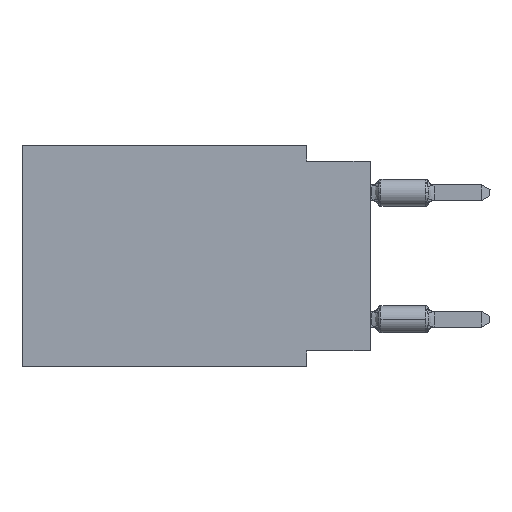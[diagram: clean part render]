
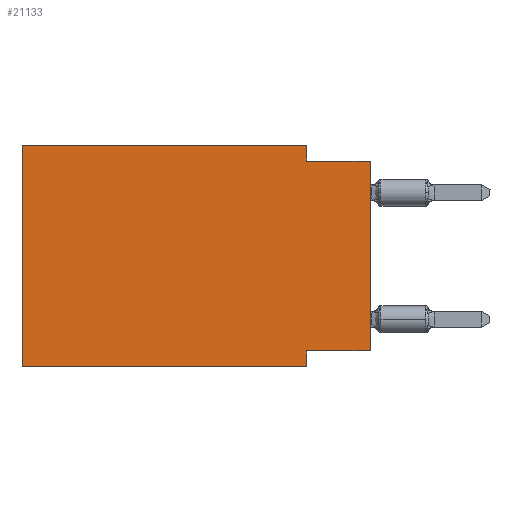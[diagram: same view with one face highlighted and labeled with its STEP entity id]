
A CAD part, left-side view. The second image highlights one B-rep face of the part: STEP entity #21133.
In plain terms, the highlighted planar face has unit normal (-1, 0, 0).
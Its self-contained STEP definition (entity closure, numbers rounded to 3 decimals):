
#241 = EDGE_CURVE ( 'NONE', #34653, #24544, #29616, .T. ) ;
#618 = CARTESIAN_POINT ( 'NONE',  ( 0., 13.97, -8.89 ) ) ;
#690 = DIRECTION ( 'NONE',  ( 0., -1., 0. ) ) ;
#969 = DIRECTION ( 'NONE',  ( 0., 0., -1. ) ) ;
#2252 = CARTESIAN_POINT ( 'NONE',  ( 0., 2.54, 0. ) ) ;
#2340 = EDGE_CURVE ( 'NONE', #28692, #20723, #17113, .T. ) ;
#2388 = CARTESIAN_POINT ( 'NONE',  ( 0., 13.97, 0. ) ) ;
#2437 = VERTEX_POINT ( 'NONE', #8050 ) ;
#2706 = VECTOR ( 'NONE', #32780, 1000. ) ;
#3138 = LINE ( 'NONE', #618, #26369 ) ;
#3163 = ORIENTED_EDGE ( 'NONE', *, *, #15992, .F. ) ;
#3321 = CARTESIAN_POINT ( 'NONE',  ( 0., 13.97, 0. ) ) ;
#4122 = AXIS2_PLACEMENT_3D ( 'NONE', #15893, #6894, #10316 ) ;
#4881 = CARTESIAN_POINT ( 'NONE',  ( 0., 13.97, 0. ) ) ;
#5258 = CARTESIAN_POINT ( 'NONE',  ( 0., 2.54, -0.635 ) ) ;
#6297 = CARTESIAN_POINT ( 'NONE',  ( 0., 2.54, -8.255 ) ) ;
#6429 = VECTOR ( 'NONE', #21536, 1000. ) ;
#6894 = DIRECTION ( 'NONE',  ( 1., 0., 0. ) ) ;
#7183 = VECTOR ( 'NONE', #969, 1000. ) ;
#7878 = LINE ( 'NONE', #2252, #2706 ) ;
#8050 = CARTESIAN_POINT ( 'NONE',  ( 0., 0., -8.255 ) ) ;
#8384 = VECTOR ( 'NONE', #26746, 1000. ) ;
#10316 = DIRECTION ( 'NONE',  ( 0., 0., -1. ) ) ;
#10370 = CARTESIAN_POINT ( 'NONE',  ( 0., 0., -8.255 ) ) ;
#10585 = CARTESIAN_POINT ( 'NONE',  ( 0., 2.54, -8.89 ) ) ;
#11467 = EDGE_CURVE ( 'NONE', #20013, #22165, #28789, .T. ) ;
#12053 = EDGE_CURVE ( 'NONE', #2437, #20723, #32335, .T. ) ;
#12486 = PLANE ( 'NONE',  #4122 ) ;
#12801 = ORIENTED_EDGE ( 'NONE', *, *, #241, .F. ) ;
#12854 = EDGE_CURVE ( 'NONE', #2437, #20013, #18299, .T. ) ;
#12998 = CARTESIAN_POINT ( 'NONE',  ( 0., 0., -0.635 ) ) ;
#14737 = ORIENTED_EDGE ( 'NONE', *, *, #34406, .T. ) ;
#15375 = VECTOR ( 'NONE', #16526, 1000. ) ;
#15893 = CARTESIAN_POINT ( 'NONE',  ( 0., 13.97, 0. ) ) ;
#15992 = EDGE_CURVE ( 'NONE', #29948, #34653, #22479, .T. ) ;
#16526 = DIRECTION ( 'NONE',  ( 0., 0., 1. ) ) ;
#16548 = ORIENTED_EDGE ( 'NONE', *, *, #2340, .F. ) ;
#17113 = LINE ( 'NONE', #23250, #28188 ) ;
#18299 = LINE ( 'NONE', #10370, #6429 ) ;
#20013 = VERTEX_POINT ( 'NONE', #6297 ) ;
#20466 = CARTESIAN_POINT ( 'NONE',  ( 0., 2.54, -8.89 ) ) ;
#20723 = VERTEX_POINT ( 'NONE', #12998 ) ;
#21133 = ADVANCED_FACE ( 'NONE', ( #34695 ), #12486, .F. ) ;
#21536 = DIRECTION ( 'NONE',  ( 0., 1., 0. ) ) ;
#22165 = VERTEX_POINT ( 'NONE', #10585 ) ;
#22479 = LINE ( 'NONE', #3321, #15375 ) ;
#22510 = ORIENTED_EDGE ( 'NONE', *, *, #12854, .F. ) ;
#23250 = CARTESIAN_POINT ( 'NONE',  ( 0., 0., -0.635 ) ) ;
#23537 = VECTOR ( 'NONE', #32503, 1000. ) ;
#24210 = CARTESIAN_POINT ( 'NONE',  ( 0., 0., 0. ) ) ;
#24488 = ORIENTED_EDGE ( 'NONE', *, *, #12053, .T. ) ;
#24544 = VERTEX_POINT ( 'NONE', #29024 ) ;
#24953 = ORIENTED_EDGE ( 'NONE', *, *, #11467, .F. ) ;
#26369 = VECTOR ( 'NONE', #30247, 1000. ) ;
#26746 = DIRECTION ( 'NONE',  ( 0., 0., 1. ) ) ;
#28188 = VECTOR ( 'NONE', #690, 1000. ) ;
#28692 = VERTEX_POINT ( 'NONE', #5258 ) ;
#28789 = LINE ( 'NONE', #20466, #7183 ) ;
#29024 = CARTESIAN_POINT ( 'NONE',  ( 0., 2.54, 0. ) ) ;
#29616 = LINE ( 'NONE', #4881, #23537 ) ;
#29948 = VERTEX_POINT ( 'NONE', #34495 ) ;
#30097 = EDGE_LOOP ( 'NONE', ( #24488, #16548, #30686, #12801, #3163, #14737, #24953, #22510 ) ) ;
#30247 = DIRECTION ( 'NONE',  ( 0., -1., 0. ) ) ;
#30686 = ORIENTED_EDGE ( 'NONE', *, *, #34294, .F. ) ;
#32335 = LINE ( 'NONE', #24210, #8384 ) ;
#32503 = DIRECTION ( 'NONE',  ( 0., -1., 0. ) ) ;
#32780 = DIRECTION ( 'NONE',  ( 0., 0., -1. ) ) ;
#34294 = EDGE_CURVE ( 'NONE', #24544, #28692, #7878, .T. ) ;
#34406 = EDGE_CURVE ( 'NONE', #29948, #22165, #3138, .T. ) ;
#34495 = CARTESIAN_POINT ( 'NONE',  ( 0., 13.97, -8.89 ) ) ;
#34653 = VERTEX_POINT ( 'NONE', #2388 ) ;
#34695 = FACE_OUTER_BOUND ( 'NONE', #30097, .T. ) ;
